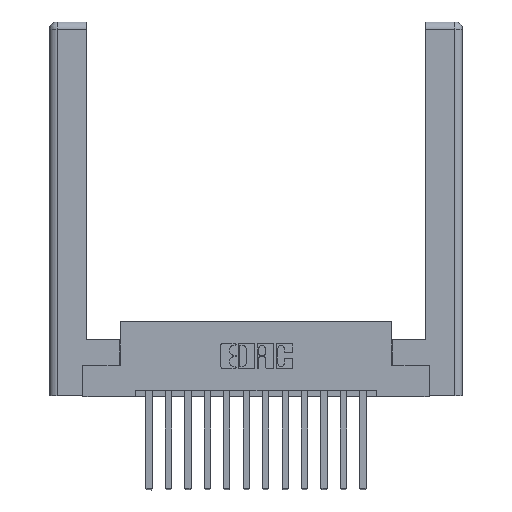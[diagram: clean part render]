
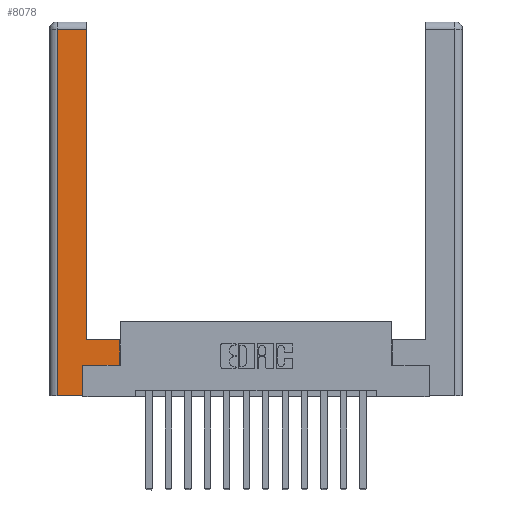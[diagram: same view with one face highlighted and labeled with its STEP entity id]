
A CAD part, top view. The second image highlights one B-rep face of the part: STEP entity #8078.
In plain terms, the highlighted planar face has unit normal (0, 0, 1).
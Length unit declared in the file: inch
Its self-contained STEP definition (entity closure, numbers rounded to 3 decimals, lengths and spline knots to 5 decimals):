
#109 = ORIENTED_EDGE ( 'NONE', *, *, #3477, .T. ) ;
#959 = VERTEX_POINT ( 'NONE', #15589 ) ;
#1072 = VERTEX_POINT ( 'NONE', #15014 ) ;
#1105 = VERTEX_POINT ( 'NONE', #4522 ) ;
#1276 = VECTOR ( 'NONE', #1642, 39.37008 ) ;
#1642 = DIRECTION ( 'NONE',  ( -1., 0., 0. ) ) ;
#1822 = DIRECTION ( 'NONE',  ( -1., 0., 0. ) ) ;
#2450 = CARTESIAN_POINT ( 'NONE',  ( 0., 0., 0. ) ) ;
#2691 = DIRECTION ( 'NONE',  ( 0., 1., 0. ) ) ;
#3101 = LINE ( 'NONE', #10946, #13922 ) ;
#3359 = CARTESIAN_POINT ( 'NONE',  ( 0.565, 0.245, 0. ) ) ;
#3377 = LINE ( 'NONE', #4317, #4505 ) ;
#3477 = EDGE_CURVE ( 'NONE', #13093, #13654, #15338, .T. ) ;
#3551 = VECTOR ( 'NONE', #3902, 39.37008 ) ;
#3902 = DIRECTION ( 'NONE',  ( 0., 1., 0. ) ) ;
#3913 = AXIS2_PLACEMENT_3D ( 'NONE', #2450, #8443, #12111 ) ;
#3928 = LINE ( 'NONE', #11145, #3551 ) ;
#4235 = EDGE_CURVE ( 'NONE', #959, #15159, #3377, .T. ) ;
#4317 = CARTESIAN_POINT ( 'NONE',  ( 0.0615, 0., 0. ) ) ;
#4505 = VECTOR ( 'NONE', #5621, 39.37008 ) ;
#4522 = CARTESIAN_POINT ( 'NONE',  ( 0.265, 0.245, 0. ) ) ;
#5621 = DIRECTION ( 'NONE',  ( 0., -1., 0. ) ) ;
#5793 = CARTESIAN_POINT ( 'NONE',  ( 0.565, 0.45, 0. ) ) ;
#6392 = ORIENTED_EDGE ( 'NONE', *, *, #13739, .T. ) ;
#6595 = PLANE ( 'NONE',  #3913 ) ;
#6976 = VERTEX_POINT ( 'NONE', #12633 ) ;
#7054 = LINE ( 'NONE', #9901, #9321 ) ;
#7238 = CARTESIAN_POINT ( 'NONE',  ( 0.0615, 0., 0. ) ) ;
#7654 = LINE ( 'NONE', #10676, #15056 ) ;
#7778 = VECTOR ( 'NONE', #14296, 39.37008 ) ;
#7948 = ORIENTED_EDGE ( 'NONE', *, *, #11581, .T. ) ;
#7990 = VERTEX_POINT ( 'NONE', #8778 ) ;
#8066 = LINE ( 'NONE', #8868, #1276 ) ;
#8078 = ADVANCED_FACE ( 'NONE', ( #13472 ), #6595, .F. ) ;
#8397 = ORIENTED_EDGE ( 'NONE', *, *, #9649, .T. ) ;
#8443 = DIRECTION ( 'NONE',  ( 0., 0., -1. ) ) ;
#8778 = CARTESIAN_POINT ( 'NONE',  ( 0.265, 0., 0. ) ) ;
#8868 = CARTESIAN_POINT ( 'NONE',  ( 0.0615, 2.94, 0. ) ) ;
#9226 = EDGE_CURVE ( 'NONE', #7990, #1105, #3928, .T. ) ;
#9321 = VECTOR ( 'NONE', #2691, 39.37008 ) ;
#9560 = DIRECTION ( 'NONE',  ( 1., 0., 0. ) ) ;
#9649 = EDGE_CURVE ( 'NONE', #1072, #959, #8066, .T. ) ;
#9901 = CARTESIAN_POINT ( 'NONE',  ( 0.565, 0.45, 0. ) ) ;
#10019 = VECTOR ( 'NONE', #1822, 39.37008 ) ;
#10214 = LINE ( 'NONE', #3359, #7778 ) ;
#10676 = CARTESIAN_POINT ( 'NONE',  ( 0.295, 3., 0. ) ) ;
#10946 = CARTESIAN_POINT ( 'NONE',  ( 0.265, 0., 0. ) ) ;
#11145 = CARTESIAN_POINT ( 'NONE',  ( 0.265, 0.245, 0. ) ) ;
#11581 = EDGE_CURVE ( 'NONE', #13654, #1072, #7654, .T. ) ;
#11776 = EDGE_CURVE ( 'NONE', #6976, #13093, #7054, .T. ) ;
#11791 = ORIENTED_EDGE ( 'NONE', *, *, #11776, .T. ) ;
#12111 = DIRECTION ( 'NONE',  ( -1., 0., 0. ) ) ;
#12149 = DIRECTION ( 'NONE',  ( 0., 1., 0. ) ) ;
#12207 = EDGE_CURVE ( 'NONE', #15159, #7990, #3101, .T. ) ;
#12361 = EDGE_LOOP ( 'NONE', ( #7948, #8397, #14057, #14831, #13436, #6392, #11791, #109 ) ) ;
#12633 = CARTESIAN_POINT ( 'NONE',  ( 0.565, 0.245, 0. ) ) ;
#13093 = VERTEX_POINT ( 'NONE', #5793 ) ;
#13160 = CARTESIAN_POINT ( 'NONE',  ( 0.295, 0.45, 0. ) ) ;
#13436 = ORIENTED_EDGE ( 'NONE', *, *, #9226, .T. ) ;
#13472 = FACE_OUTER_BOUND ( 'NONE', #12361, .T. ) ;
#13654 = VERTEX_POINT ( 'NONE', #13160 ) ;
#13739 = EDGE_CURVE ( 'NONE', #1105, #6976, #10214, .T. ) ;
#13922 = VECTOR ( 'NONE', #9560, 39.37008 ) ;
#14057 = ORIENTED_EDGE ( 'NONE', *, *, #4235, .T. ) ;
#14296 = DIRECTION ( 'NONE',  ( 1., 0., 0. ) ) ;
#14831 = ORIENTED_EDGE ( 'NONE', *, *, #12207, .T. ) ;
#15014 = CARTESIAN_POINT ( 'NONE',  ( 0.295, 2.94, 0. ) ) ;
#15056 = VECTOR ( 'NONE', #12149, 39.37008 ) ;
#15063 = CARTESIAN_POINT ( 'NONE',  ( 0.295, 0.45, 0. ) ) ;
#15159 = VERTEX_POINT ( 'NONE', #7238 ) ;
#15338 = LINE ( 'NONE', #15063, #10019 ) ;
#15589 = CARTESIAN_POINT ( 'NONE',  ( 0.0615, 2.94, 0. ) ) ;
